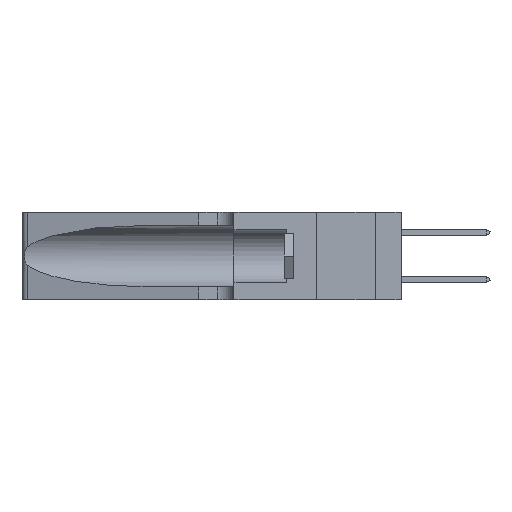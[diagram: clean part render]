
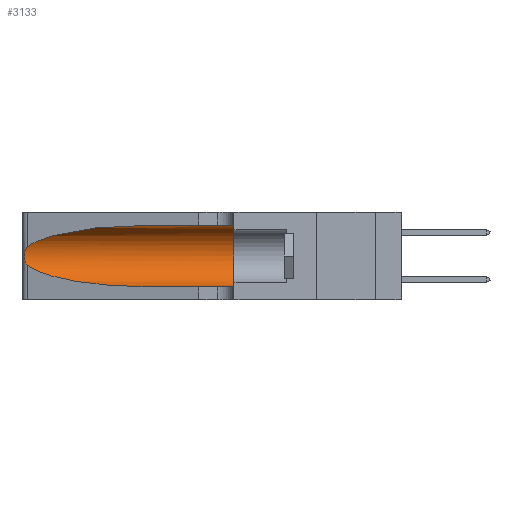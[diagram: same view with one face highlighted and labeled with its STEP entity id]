
A CAD part, left-side view. The second image highlights one B-rep face of the part: STEP entity #3133.
In plain terms, the highlighted cylindrical face has radius 3.308 mm (diameter 6.617 mm), a partial arc.
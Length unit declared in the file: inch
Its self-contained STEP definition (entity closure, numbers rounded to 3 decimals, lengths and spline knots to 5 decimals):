
#449 = CARTESIAN_POINT ( 'NONE',  ( 0.1305, 0.35, 0.05475 ) ) ;
#520 = CARTESIAN_POINT ( 'NONE',  ( 0.25555, 1.22994, 0.2215 ) ) ;
#715 =( BOUNDED_CURVE ( )  B_SPLINE_CURVE ( 3, ( #8207, #26366, #17336, #3724 ),
 .UNSPECIFIED., .F., .F. ) 
 B_SPLINE_CURVE_WITH_KNOTS ( ( 4, 4 ),
 ( 3.44316, 4.71239 ),
 .UNSPECIFIED. ) 
 CURVE ( )  GEOMETRIC_REPRESENTATION_ITEM ( )  RATIONAL_B_SPLINE_CURVE ( ( 1., 0.87, 0.87, 1. ) ) 
 REPRESENTATION_ITEM ( '' )  );
#1893 = CARTESIAN_POINT ( 'NONE',  ( 0.26075, 1.23896, 0.19203 ) ) ;
#2168 = ORIENTED_EDGE ( 'NONE', *, *, #3399, .F. ) ;
#2299 = CARTESIAN_POINT ( 'NONE',  ( 0.1305, 0.72297, 0.31525 ) ) ;
#2580 = EDGE_CURVE ( 'NONE', #17799, #6665, #6068, .T. ) ;
#2662 = AXIS2_PLACEMENT_3D ( 'NONE', #27040, #26940, #13750 ) ;
#2821 = CARTESIAN_POINT ( 'NONE',  ( 0.25487, 1.22718, 0.22369 ) ) ;
#3133 = ADVANCED_FACE ( 'NONE', ( #7573 ), #6854, .F. ) ;
#3237 = CARTESIAN_POINT ( 'NONE',  ( 0.1305, 0.35, 0.31525 ) ) ;
#3399 = EDGE_CURVE ( 'NONE', #25157, #10120, #21066, .T. ) ;
#3724 = CARTESIAN_POINT ( 'NONE',  ( 0.1305, 0.72297, 0.05475 ) ) ;
#4447 = CARTESIAN_POINT ( 'NONE',  ( 0.25487, 1.22718, 0.22369 ) ) ;
#4549 = EDGE_CURVE ( 'NONE', #6665, #24110, #715, .T. ) ;
#4880 = CARTESIAN_POINT ( 'NONE',  ( 0.25789, 1.23486, 0.15765 ) ) ;
#6068 = B_SPLINE_CURVE_WITH_KNOTS ( 'NONE', 3,
 ( #28070, #520, #16446, #20395, #6802, #15553, #1893, #8805, #24673, #29232, #4880, #23043, #11768, #27638 ),
 .UNSPECIFIED., .F., .F.,
 ( 4, 2, 2, 2, 2, 2, 4 ),
 ( 0., 0.00027, 0.00053, 0.00107, 0.0016, 0.00187, 0.00214 ),
 .UNSPECIFIED. ) ;
#6665 = VERTEX_POINT ( 'NONE', #16554 ) ;
#6802 = CARTESIAN_POINT ( 'NONE',  ( 0.25854, 1.2359, 0.20912 ) ) ;
#6854 = CYLINDRICAL_SURFACE ( 'NONE', #22520, 0.13025 ) ;
#7206 = EDGE_CURVE ( 'NONE', #24110, #10120, #23578, .T. ) ;
#7573 = FACE_OUTER_BOUND ( 'NONE', #28408, .T. ) ;
#8157 = CARTESIAN_POINT ( 'NONE',  ( 0.1305, 1.61858, 0.31525 ) ) ;
#8207 = CARTESIAN_POINT ( 'NONE',  ( 0.25487, 1.22718, 0.14631 ) ) ;
#8805 = CARTESIAN_POINT ( 'NONE',  ( 0.26075, 1.23896, 0.178 ) ) ;
#8980 = CARTESIAN_POINT ( 'NONE',  ( 0.1305, 0.72297, 0.05475 ) ) ;
#10120 = VERTEX_POINT ( 'NONE', #449 ) ;
#11768 = CARTESIAN_POINT ( 'NONE',  ( 0.25555, 1.22993, 0.14849 ) ) ;
#13736 = ORIENTED_EDGE ( 'NONE', *, *, #22455, .F. ) ;
#13750 = DIRECTION ( 'NONE',  ( 0., 0., 1. ) ) ;
#15318 = CARTESIAN_POINT ( 'NONE',  ( 0.1305, 1.61858, 0.05475 ) ) ;
#15553 = CARTESIAN_POINT ( 'NONE',  ( 0.26018, 1.23835, 0.19895 ) ) ;
#16396 =( BOUNDED_CURVE ( )  B_SPLINE_CURVE ( 3, ( #2299, #20227, #20521, #4447 ),
 .UNSPECIFIED., .F., .T. ) 
 B_SPLINE_CURVE_WITH_KNOTS ( ( 4, 4 ),
 ( 1.5708, 2.84003 ),
 .UNSPECIFIED. ) 
 CURVE ( )  GEOMETRIC_REPRESENTATION_ITEM ( )  RATIONAL_B_SPLINE_CURVE ( ( 1., 0.87, 0.87, 1. ) ) 
 REPRESENTATION_ITEM ( '' )  );
#16446 = CARTESIAN_POINT ( 'NONE',  ( 0.25639, 1.23184, 0.21858 ) ) ;
#16554 = CARTESIAN_POINT ( 'NONE',  ( 0.25487, 1.22718, 0.14631 ) ) ;
#16676 = EDGE_CURVE ( 'NONE', #25128, #17799, #16396, .T. ) ;
#17336 = CARTESIAN_POINT ( 'NONE',  ( 0.18966, 0.96281, 0.05475 ) ) ;
#17799 = VERTEX_POINT ( 'NONE', #2821 ) ;
#18955 = CARTESIAN_POINT ( 'NONE',  ( 0.1305, 0.72297, 0.31525 ) ) ;
#20227 = CARTESIAN_POINT ( 'NONE',  ( 0.18966, 0.96281, 0.31525 ) ) ;
#20263 = ORIENTED_EDGE ( 'NONE', *, *, #7206, .T. ) ;
#20395 = CARTESIAN_POINT ( 'NONE',  ( 0.25787, 1.23484, 0.2124 ) ) ;
#20521 = CARTESIAN_POINT ( 'NONE',  ( 0.2373, 1.15595, 0.28018 ) ) ;
#20540 = DIRECTION ( 'NONE',  ( 0., -1., 0. ) ) ;
#20637 = DIRECTION ( 'NONE',  ( 0., 0., -1. ) ) ;
#21066 = CIRCLE ( 'NONE', #2662, 0.13025 ) ;
#22105 = ORIENTED_EDGE ( 'NONE', *, *, #2580, .T. ) ;
#22455 = EDGE_CURVE ( 'NONE', #25128, #25157, #26320, .T. ) ;
#22520 = AXIS2_PLACEMENT_3D ( 'NONE', #24340, #20540, #20637 ) ;
#22905 = DIRECTION ( 'NONE',  ( 0., -1., 0. ) ) ;
#23043 = CARTESIAN_POINT ( 'NONE',  ( 0.25639, 1.23186, 0.15144 ) ) ;
#23578 = LINE ( 'NONE', #15318, #25721 ) ;
#24110 = VERTEX_POINT ( 'NONE', #8980 ) ;
#24170 = VECTOR ( 'NONE', #26203, 39.37008 ) ;
#24340 = CARTESIAN_POINT ( 'NONE',  ( 0.1305, 1.61858, 0.185 ) ) ;
#24485 = ORIENTED_EDGE ( 'NONE', *, *, #16676, .T. ) ;
#24673 = CARTESIAN_POINT ( 'NONE',  ( 0.26017, 1.23833, 0.17102 ) ) ;
#25128 = VERTEX_POINT ( 'NONE', #18955 ) ;
#25157 = VERTEX_POINT ( 'NONE', #3237 ) ;
#25721 = VECTOR ( 'NONE', #22905, 39.37008 ) ;
#25758 = ORIENTED_EDGE ( 'NONE', *, *, #4549, .T. ) ;
#26203 = DIRECTION ( 'NONE',  ( 0., -1., 0. ) ) ;
#26320 = LINE ( 'NONE', #8157, #24170 ) ;
#26366 = CARTESIAN_POINT ( 'NONE',  ( 0.2373, 1.15595, 0.08982 ) ) ;
#26940 = DIRECTION ( 'NONE',  ( 0., 1., 0. ) ) ;
#27040 = CARTESIAN_POINT ( 'NONE',  ( 0.1305, 0.35, 0.185 ) ) ;
#27638 = CARTESIAN_POINT ( 'NONE',  ( 0.25487, 1.22718, 0.14631 ) ) ;
#28070 = CARTESIAN_POINT ( 'NONE',  ( 0.25487, 1.22718, 0.22369 ) ) ;
#28408 = EDGE_LOOP ( 'NONE', ( #24485, #22105, #25758, #20263, #2168, #13736 ) ) ;
#29232 = CARTESIAN_POINT ( 'NONE',  ( 0.25856, 1.23593, 0.16098 ) ) ;
